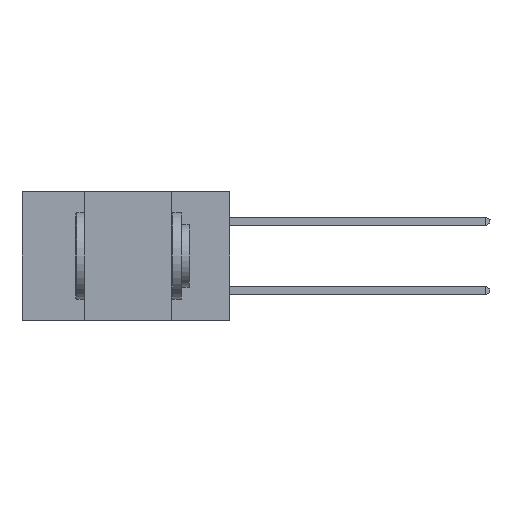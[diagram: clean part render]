
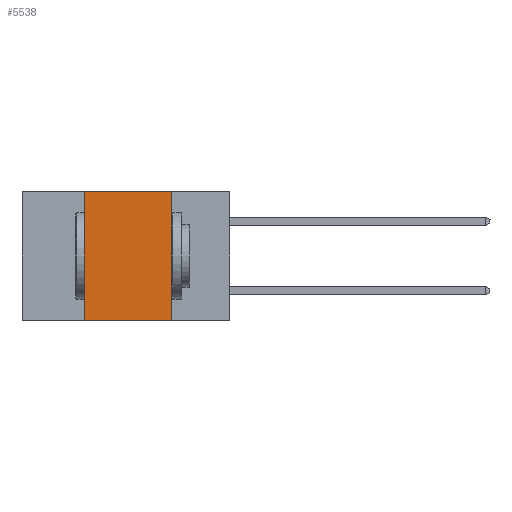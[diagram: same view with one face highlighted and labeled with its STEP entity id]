
A CAD part, left-side view. The second image highlights one B-rep face of the part: STEP entity #5538.
In plain terms, the highlighted planar face has unit normal (-1, 0, 0).
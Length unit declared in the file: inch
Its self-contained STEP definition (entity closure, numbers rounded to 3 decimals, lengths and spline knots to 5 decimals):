
#478 = VERTEX_POINT ( 'NONE', #19480 ) ;
#479 = EDGE_CURVE ( 'NONE', #21295, #478, #7831, .T. ) ;
#3140 = CARTESIAN_POINT ( 'NONE',  ( 0., 0.17, -0.37 ) ) ;
#4375 = CARTESIAN_POINT ( 'NONE',  ( 0., 0.42, 0. ) ) ;
#5538 = ADVANCED_FACE ( 'NONE', ( #5691 ), #17313, .F. ) ;
#5691 = FACE_OUTER_BOUND ( 'NONE', #7727, .T. ) ;
#6181 = DIRECTION ( 'NONE',  ( 0., -1., 0. ) ) ;
#6314 = VERTEX_POINT ( 'NONE', #3140 ) ;
#7727 = EDGE_LOOP ( 'NONE', ( #18124, #13723, #21522, #12662 ) ) ;
#7768 = VECTOR ( 'NONE', #9213, 39.37008 ) ;
#7831 = LINE ( 'NONE', #9482, #12615 ) ;
#8781 = VERTEX_POINT ( 'NONE', #21653 ) ;
#8802 = CARTESIAN_POINT ( 'NONE',  ( 0., 0.6, -0.37 ) ) ;
#8876 = DIRECTION ( 'NONE',  ( 1., 0., 0. ) ) ;
#8931 = EDGE_CURVE ( 'NONE', #8781, #6314, #20758, .T. ) ;
#9213 = DIRECTION ( 'NONE',  ( 0., -1., 0. ) ) ;
#9482 = CARTESIAN_POINT ( 'NONE',  ( 0., 0.6, 0. ) ) ;
#10956 = EDGE_CURVE ( 'NONE', #478, #6314, #19292, .T. ) ;
#11065 = CARTESIAN_POINT ( 'NONE',  ( 0., 0.17, -0.37 ) ) ;
#12615 = VECTOR ( 'NONE', #6181, 39.37008 ) ;
#12662 = ORIENTED_EDGE ( 'NONE', *, *, #8931, .T. ) ;
#13723 = ORIENTED_EDGE ( 'NONE', *, *, #479, .F. ) ;
#13771 = VECTOR ( 'NONE', #14567, 39.37008 ) ;
#14549 = LINE ( 'NONE', #17733, #19830 ) ;
#14567 = DIRECTION ( 'NONE',  ( 0., 0., -1. ) ) ;
#15977 = DIRECTION ( 'NONE',  ( 0., 0., 1. ) ) ;
#16897 = EDGE_CURVE ( 'NONE', #8781, #21295, #14549, .T. ) ;
#17105 = DIRECTION ( 'NONE',  ( 0., 0., -1. ) ) ;
#17157 = AXIS2_PLACEMENT_3D ( 'NONE', #20837, #8876, #17105 ) ;
#17313 = PLANE ( 'NONE',  #17157 ) ;
#17733 = CARTESIAN_POINT ( 'NONE',  ( 0., 0.42, -0.37 ) ) ;
#18124 = ORIENTED_EDGE ( 'NONE', *, *, #10956, .F. ) ;
#19292 = LINE ( 'NONE', #11065, #13771 ) ;
#19480 = CARTESIAN_POINT ( 'NONE',  ( 0., 0.17, 0. ) ) ;
#19830 = VECTOR ( 'NONE', #15977, 39.37008 ) ;
#20758 = LINE ( 'NONE', #8802, #7768 ) ;
#20837 = CARTESIAN_POINT ( 'NONE',  ( 0., 0.6, 0. ) ) ;
#21295 = VERTEX_POINT ( 'NONE', #4375 ) ;
#21522 = ORIENTED_EDGE ( 'NONE', *, *, #16897, .F. ) ;
#21653 = CARTESIAN_POINT ( 'NONE',  ( 0., 0.42, -0.37 ) ) ;
